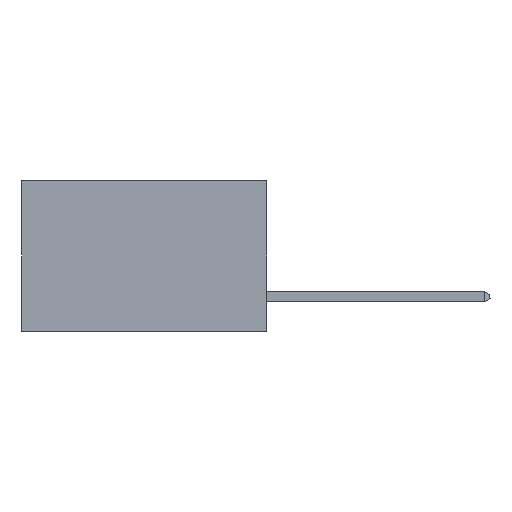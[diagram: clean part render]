
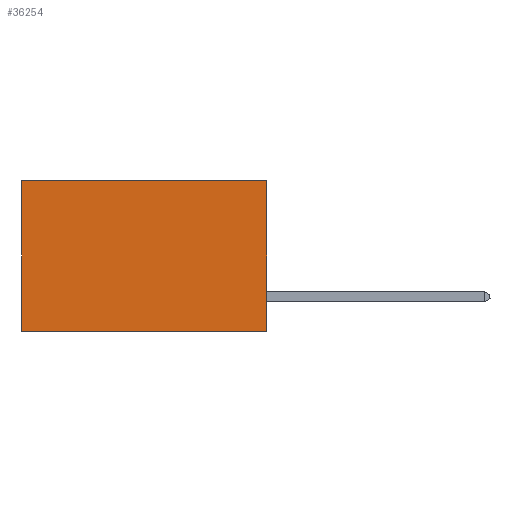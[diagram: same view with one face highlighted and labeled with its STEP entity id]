
A CAD part, left-side view. The second image highlights one B-rep face of the part: STEP entity #36254.
In plain terms, the highlighted planar face has unit normal (-1, 0, 0).
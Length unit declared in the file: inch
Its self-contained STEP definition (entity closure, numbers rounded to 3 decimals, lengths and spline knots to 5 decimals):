
#1214 = VECTOR ( 'NONE', #1532, 39.37008 ) ;
#1532 = DIRECTION ( 'NONE',  ( 0., 0., -1. ) ) ;
#1789 = EDGE_LOOP ( 'NONE', ( #2228, #38874, #14917, #24258 ) ) ;
#1808 = DIRECTION ( 'NONE',  ( 0., 0., -1. ) ) ;
#2221 = LINE ( 'NONE', #5061, #1214 ) ;
#2228 = ORIENTED_EDGE ( 'NONE', *, *, #36243, .T. ) ;
#2378 = EDGE_CURVE ( 'NONE', #33415, #8883, #13197, .T. ) ;
#2475 = CARTESIAN_POINT ( 'NONE',  ( 0.2875, 0., 0. ) ) ;
#2762 = DIRECTION ( 'NONE',  ( 0., 0., -1. ) ) ;
#3257 = FACE_OUTER_BOUND ( 'NONE', #1789, .T. ) ;
#5061 = CARTESIAN_POINT ( 'NONE',  ( 0.2875, 0.6, 0. ) ) ;
#8733 = VERTEX_POINT ( 'NONE', #23787 ) ;
#8883 = VERTEX_POINT ( 'NONE', #30063 ) ;
#9534 = CARTESIAN_POINT ( 'NONE',  ( 0.2875, 0.6, -0.37 ) ) ;
#9998 = EDGE_CURVE ( 'NONE', #8883, #17771, #32125, .T. ) ;
#11626 = DIRECTION ( 'NONE',  ( 0., 1., 0. ) ) ;
#13197 = LINE ( 'NONE', #2475, #18216 ) ;
#14917 = ORIENTED_EDGE ( 'NONE', *, *, #2378, .F. ) ;
#16983 = VECTOR ( 'NONE', #18233, 39.37008 ) ;
#17771 = VERTEX_POINT ( 'NONE', #9534 ) ;
#18216 = VECTOR ( 'NONE', #2762, 39.37008 ) ;
#18233 = DIRECTION ( 'NONE',  ( 0., 1., 0. ) ) ;
#21310 = EDGE_CURVE ( 'NONE', #33415, #8733, #29123, .T. ) ;
#23617 = CARTESIAN_POINT ( 'NONE',  ( 0.2875, 0., 0. ) ) ;
#23787 = CARTESIAN_POINT ( 'NONE',  ( 0.2875, 0.6, 0. ) ) ;
#24258 = ORIENTED_EDGE ( 'NONE', *, *, #21310, .T. ) ;
#24500 = DIRECTION ( 'NONE',  ( 1., 0., 0. ) ) ;
#29123 = LINE ( 'NONE', #31672, #16983 ) ;
#30063 = CARTESIAN_POINT ( 'NONE',  ( 0.2875, 0., -0.37 ) ) ;
#30873 = CARTESIAN_POINT ( 'NONE',  ( 0.2875, 0., 0. ) ) ;
#30931 = CARTESIAN_POINT ( 'NONE',  ( 0.2875, 0., -0.37 ) ) ;
#31672 = CARTESIAN_POINT ( 'NONE',  ( 0.2875, 0., 0. ) ) ;
#32125 = LINE ( 'NONE', #30931, #41751 ) ;
#33415 = VERTEX_POINT ( 'NONE', #23617 ) ;
#33838 = PLANE ( 'NONE',  #34794 ) ;
#34794 = AXIS2_PLACEMENT_3D ( 'NONE', #30873, #24500, #1808 ) ;
#36243 = EDGE_CURVE ( 'NONE', #8733, #17771, #2221, .T. ) ;
#36254 = ADVANCED_FACE ( 'NONE', ( #3257 ), #33838, .F. ) ;
#38874 = ORIENTED_EDGE ( 'NONE', *, *, #9998, .F. ) ;
#41751 = VECTOR ( 'NONE', #11626, 39.37008 ) ;
